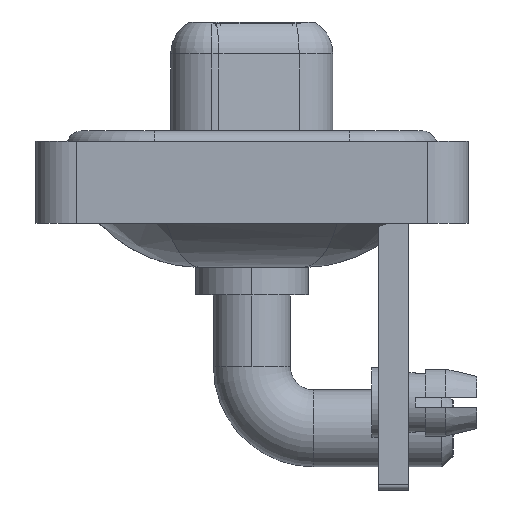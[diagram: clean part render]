
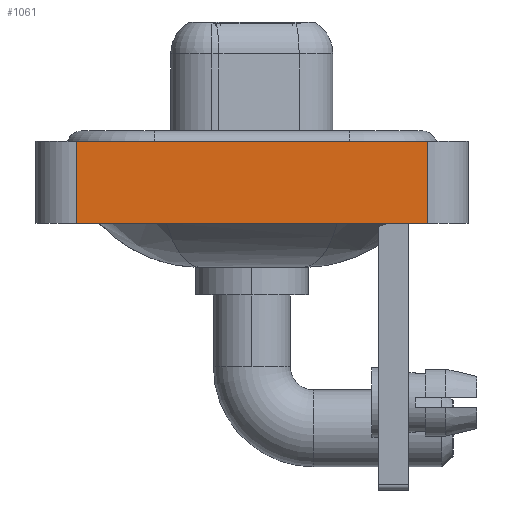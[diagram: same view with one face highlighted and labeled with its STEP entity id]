
A CAD part, left-side view. The second image highlights one B-rep face of the part: STEP entity #1061.
In plain terms, the highlighted planar face has unit normal (-1, 0, 0).
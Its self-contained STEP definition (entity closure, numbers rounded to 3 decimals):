
#771 = FACE_OUTER_BOUND ( 'NONE', #6383, .T. ) ;
#814 = DIRECTION ( 'NONE',  ( 0., -1., 0. ) ) ;
#1061 = ADVANCED_FACE ( 'NONE', ( #771 ), #12439, .T. ) ;
#1803 = VERTEX_POINT ( 'NONE', #12005 ) ;
#2269 = CARTESIAN_POINT ( 'NONE',  ( -7.25, 8.55, -3.6 ) ) ;
#2588 = VECTOR ( 'NONE', #814, 1000. ) ;
#2687 = CARTESIAN_POINT ( 'NONE',  ( -7.25, -8.55, -3.6 ) ) ;
#2732 = CARTESIAN_POINT ( 'NONE',  ( -7.25, -8.55, -3.6 ) ) ;
#3515 = VECTOR ( 'NONE', #13263, 1000. ) ;
#4030 = LINE ( 'NONE', #14144, #2588 ) ;
#4040 = LINE ( 'NONE', #5814, #3515 ) ;
#4889 = VERTEX_POINT ( 'NONE', #14708 ) ;
#5076 = DIRECTION ( 'NONE',  ( 0., 0., 1. ) ) ;
#5565 = CARTESIAN_POINT ( 'NONE',  ( -7.25, 8.55, 0.4 ) ) ;
#5814 = CARTESIAN_POINT ( 'NONE',  ( -7.25, -8.55, -3.6 ) ) ;
#6108 = EDGE_CURVE ( 'NONE', #17685, #4889, #4030, .T. ) ;
#6383 = EDGE_LOOP ( 'NONE', ( #13651, #16143, #14447, #8816 ) ) ;
#8676 = DIRECTION ( 'NONE',  ( 0., -1., 0. ) ) ;
#8816 = ORIENTED_EDGE ( 'NONE', *, *, #9055, .T. ) ;
#9055 = EDGE_CURVE ( 'NONE', #1803, #9958, #16139, .T. ) ;
#9430 = EDGE_CURVE ( 'NONE', #1803, #17685, #19030, .T. ) ;
#9958 = VERTEX_POINT ( 'NONE', #2732 ) ;
#11349 = CARTESIAN_POINT ( 'NONE',  ( -7.25, -8.55, -3.6 ) ) ;
#11650 = EDGE_CURVE ( 'NONE', #9958, #4889, #4040, .T. ) ;
#12005 = CARTESIAN_POINT ( 'NONE',  ( -7.25, 8.55, -3.6 ) ) ;
#12439 = PLANE ( 'NONE',  #13932 ) ;
#12623 = DIRECTION ( 'NONE',  ( -1., 0., 0. ) ) ;
#13153 = DIRECTION ( 'NONE',  ( 0., 0., 1. ) ) ;
#13258 = VECTOR ( 'NONE', #13153, 1000. ) ;
#13263 = DIRECTION ( 'NONE',  ( 0., 0., 1. ) ) ;
#13651 = ORIENTED_EDGE ( 'NONE', *, *, #11650, .T. ) ;
#13932 = AXIS2_PLACEMENT_3D ( 'NONE', #11349, #12623, #5076 ) ;
#14144 = CARTESIAN_POINT ( 'NONE',  ( -7.25, -8.55, 0.4 ) ) ;
#14447 = ORIENTED_EDGE ( 'NONE', *, *, #9430, .F. ) ;
#14708 = CARTESIAN_POINT ( 'NONE',  ( -7.25, -8.55, 0.4 ) ) ;
#16139 = LINE ( 'NONE', #2687, #16981 ) ;
#16143 = ORIENTED_EDGE ( 'NONE', *, *, #6108, .F. ) ;
#16981 = VECTOR ( 'NONE', #8676, 1000. ) ;
#17685 = VERTEX_POINT ( 'NONE', #5565 ) ;
#19030 = LINE ( 'NONE', #2269, #13258 ) ;
